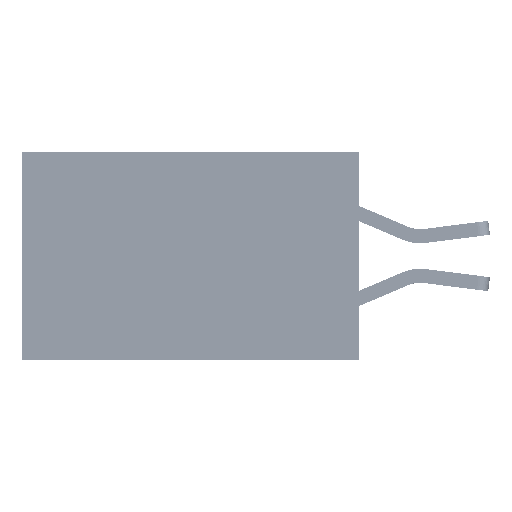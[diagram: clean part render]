
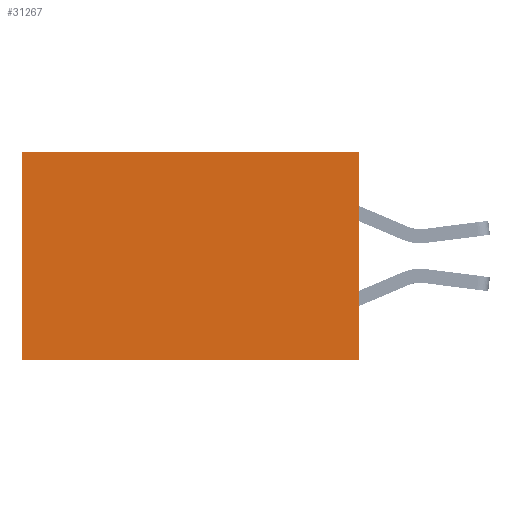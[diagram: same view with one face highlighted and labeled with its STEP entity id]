
A CAD part, left-side view. The second image highlights one B-rep face of the part: STEP entity #31267.
In plain terms, the highlighted planar face has unit normal (-1, 0, 0).
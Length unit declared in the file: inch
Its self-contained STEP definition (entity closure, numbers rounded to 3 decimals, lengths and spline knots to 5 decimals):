
#553 = CARTESIAN_POINT ( 'NONE',  ( 0.2875, 0., -0.37 ) ) ;
#875 = ORIENTED_EDGE ( 'NONE', *, *, #26965, .F. ) ;
#1091 = EDGE_CURVE ( 'NONE', #18289, #28387, #35773, .T. ) ;
#1237 = VECTOR ( 'NONE', #15887, 39.37008 ) ;
#1278 = CARTESIAN_POINT ( 'NONE',  ( 0.2875, 0., 0. ) ) ;
#1494 = DIRECTION ( 'NONE',  ( 1., 0., 0. ) ) ;
#3389 = AXIS2_PLACEMENT_3D ( 'NONE', #13159, #1494, #9330 ) ;
#5425 = VERTEX_POINT ( 'NONE', #11115 ) ;
#5671 = LINE ( 'NONE', #25473, #33075 ) ;
#6032 = CARTESIAN_POINT ( 'NONE',  ( 0.2875, 0.6, -0.37 ) ) ;
#9139 = DIRECTION ( 'NONE',  ( 0., 0., -1. ) ) ;
#9330 = DIRECTION ( 'NONE',  ( 0., 0., -1. ) ) ;
#10074 = ORIENTED_EDGE ( 'NONE', *, *, #42772, .T. ) ;
#11115 = CARTESIAN_POINT ( 'NONE',  ( 0.2875, 0.6, 0. ) ) ;
#11469 = ORIENTED_EDGE ( 'NONE', *, *, #44367, .T. ) ;
#13098 = ORIENTED_EDGE ( 'NONE', *, *, #1091, .F. ) ;
#13159 = CARTESIAN_POINT ( 'NONE',  ( 0.2875, 0., 0. ) ) ;
#14234 = FACE_OUTER_BOUND ( 'NONE', #23610, .T. ) ;
#15887 = DIRECTION ( 'NONE',  ( 0., 1., 0. ) ) ;
#17767 = VECTOR ( 'NONE', #9139, 39.37008 ) ;
#18289 = VERTEX_POINT ( 'NONE', #553 ) ;
#21153 = DIRECTION ( 'NONE',  ( 0., 0., -1. ) ) ;
#23610 = EDGE_LOOP ( 'NONE', ( #10074, #13098, #875, #11469 ) ) ;
#25473 = CARTESIAN_POINT ( 'NONE',  ( 0.2875, 0.6, 0. ) ) ;
#26965 = EDGE_CURVE ( 'NONE', #48412, #18289, #30824, .T. ) ;
#27589 = DIRECTION ( 'NONE',  ( 0., 1., 0. ) ) ;
#28106 = CARTESIAN_POINT ( 'NONE',  ( 0.2875, 0., 0. ) ) ;
#28387 = VERTEX_POINT ( 'NONE', #6032 ) ;
#29349 = VECTOR ( 'NONE', #27589, 39.37008 ) ;
#30824 = LINE ( 'NONE', #28106, #17767 ) ;
#31267 = ADVANCED_FACE ( 'NONE', ( #14234 ), #39438, .F. ) ;
#33075 = VECTOR ( 'NONE', #21153, 39.37008 ) ;
#35773 = LINE ( 'NONE', #46156, #1237 ) ;
#39438 = PLANE ( 'NONE',  #3389 ) ;
#42772 = EDGE_CURVE ( 'NONE', #5425, #28387, #5671, .T. ) ;
#44367 = EDGE_CURVE ( 'NONE', #48412, #5425, #44809, .T. ) ;
#44809 = LINE ( 'NONE', #1278, #29349 ) ;
#45706 = CARTESIAN_POINT ( 'NONE',  ( 0.2875, 0., 0. ) ) ;
#46156 = CARTESIAN_POINT ( 'NONE',  ( 0.2875, 0., -0.37 ) ) ;
#48412 = VERTEX_POINT ( 'NONE', #45706 ) ;
